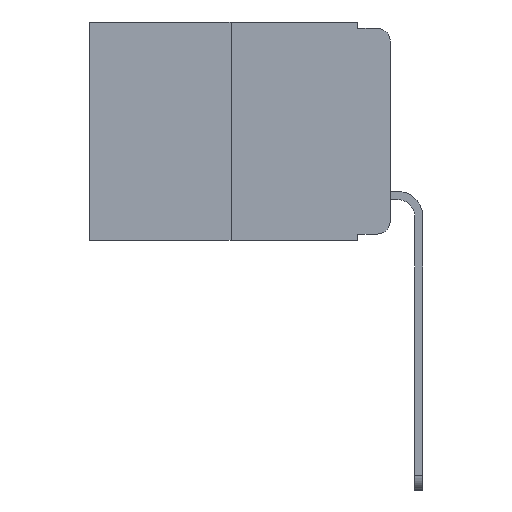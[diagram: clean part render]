
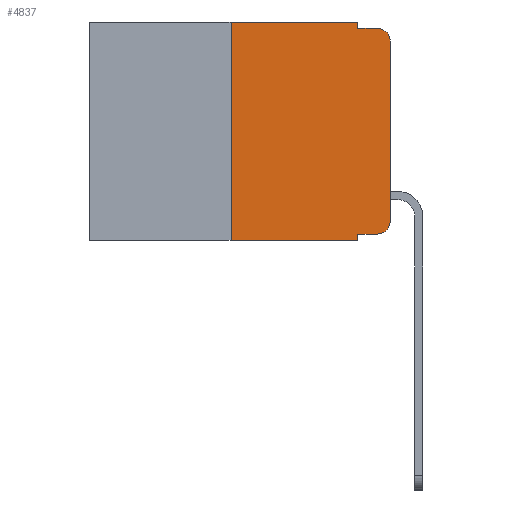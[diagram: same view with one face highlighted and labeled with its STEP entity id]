
A CAD part, left-side view. The second image highlights one B-rep face of the part: STEP entity #4837.
In plain terms, the highlighted planar face has unit normal (-1, 0, 0).
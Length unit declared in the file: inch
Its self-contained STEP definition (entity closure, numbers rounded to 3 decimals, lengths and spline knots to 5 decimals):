
#92 = CARTESIAN_POINT ( 'NONE',  ( 0., 0.02, -0.313 ) ) ;
#357 = DIRECTION ( 'NONE',  ( -1., 0., 0. ) ) ;
#649 = EDGE_CURVE ( 'NONE', #11194, #3836, #3087, .T. ) ;
#843 = CIRCLE ( 'NONE', #3029, 0.02 ) ;
#900 = CARTESIAN_POINT ( 'NONE',  ( 0., 0., -0.313 ) ) ;
#951 = CARTESIAN_POINT ( 'NONE',  ( 0., 0.051, -0.01 ) ) ;
#1226 = VECTOR ( 'NONE', #12074, 39.37008 ) ;
#1256 = LINE ( 'NONE', #2487, #8722 ) ;
#1685 = AXIS2_PLACEMENT_3D ( 'NONE', #9962, #4475, #8779 ) ;
#1732 = LINE ( 'NONE', #2476, #4293 ) ;
#1892 = CARTESIAN_POINT ( 'NONE',  ( 0., 0., -0.03 ) ) ;
#1922 = LINE ( 'NONE', #12466, #9677 ) ;
#2108 = DIRECTION ( 'NONE',  ( -1., 0., 0. ) ) ;
#2287 = ORIENTED_EDGE ( 'NONE', *, *, #12349, .F. ) ;
#2432 = ORIENTED_EDGE ( 'NONE', *, *, #12384, .F. ) ;
#2476 = CARTESIAN_POINT ( 'NONE',  ( 0., 0.051, -0.333 ) ) ;
#2487 = CARTESIAN_POINT ( 'NONE',  ( 0., 0.051, 0. ) ) ;
#2588 = CIRCLE ( 'NONE', #11765, 0.02 ) ;
#2600 = ORIENTED_EDGE ( 'NONE', *, *, #11514, .F. ) ;
#2742 = VECTOR ( 'NONE', #11522, 39.37008 ) ;
#2748 = ORIENTED_EDGE ( 'NONE', *, *, #10290, .T. ) ;
#2786 = EDGE_CURVE ( 'NONE', #12239, #5759, #843, .T. ) ;
#2811 = CARTESIAN_POINT ( 'NONE',  ( 0., 0.051, 0. ) ) ;
#2853 = DIRECTION ( 'NONE',  ( 0., -1., 0. ) ) ;
#2943 = ORIENTED_EDGE ( 'NONE', *, *, #6075, .T. ) ;
#3029 = AXIS2_PLACEMENT_3D ( 'NONE', #92, #357, #11572 ) ;
#3087 = LINE ( 'NONE', #10146, #10669 ) ;
#3102 = DIRECTION ( 'NONE',  ( 0., 0., -1. ) ) ;
#3784 = VERTEX_POINT ( 'NONE', #7944 ) ;
#3836 = VERTEX_POINT ( 'NONE', #10761 ) ;
#4117 = VECTOR ( 'NONE', #11931, 39.37008 ) ;
#4293 = VECTOR ( 'NONE', #11411, 39.37008 ) ;
#4377 = CARTESIAN_POINT ( 'NONE',  ( 0., 0.473, 0. ) ) ;
#4475 = DIRECTION ( 'NONE',  ( 1., 0., 0. ) ) ;
#4742 = VECTOR ( 'NONE', #10235, 39.37008 ) ;
#4775 = CARTESIAN_POINT ( 'NONE',  ( 0., 0.25, 0. ) ) ;
#4812 = VERTEX_POINT ( 'NONE', #1892 ) ;
#4837 = ADVANCED_FACE ( 'NONE', ( #12047 ), #11092, .F. ) ;
#5175 = VERTEX_POINT ( 'NONE', #7815 ) ;
#5425 = CARTESIAN_POINT ( 'NONE',  ( 0., 0.051, 0. ) ) ;
#5643 = VERTEX_POINT ( 'NONE', #7412 ) ;
#5759 = VERTEX_POINT ( 'NONE', #900 ) ;
#6075 = EDGE_CURVE ( 'NONE', #5759, #4812, #1922, .T. ) ;
#6651 = EDGE_CURVE ( 'NONE', #3784, #3836, #1256, .T. ) ;
#6743 = LINE ( 'NONE', #951, #4117 ) ;
#7152 = ORIENTED_EDGE ( 'NONE', *, *, #8594, .F. ) ;
#7174 = ORIENTED_EDGE ( 'NONE', *, *, #649, .T. ) ;
#7412 = CARTESIAN_POINT ( 'NONE',  ( 0., 0.051, -0.01 ) ) ;
#7558 = ORIENTED_EDGE ( 'NONE', *, *, #10623, .T. ) ;
#7672 = ORIENTED_EDGE ( 'NONE', *, *, #6651, .F. ) ;
#7815 = CARTESIAN_POINT ( 'NONE',  ( 0., 0.25, 0. ) ) ;
#7944 = CARTESIAN_POINT ( 'NONE',  ( 0., 0.051, -0.333 ) ) ;
#7966 = ORIENTED_EDGE ( 'NONE', *, *, #2786, .T. ) ;
#8213 = CARTESIAN_POINT ( 'NONE',  ( 0., 0.02, -0.03 ) ) ;
#8594 = EDGE_CURVE ( 'NONE', #11194, #5175, #9331, .T. ) ;
#8722 = VECTOR ( 'NONE', #3102, 39.37008 ) ;
#8779 = DIRECTION ( 'NONE',  ( 0., 0., -1. ) ) ;
#8876 = DIRECTION ( 'NONE',  ( 0., 0., 1. ) ) ;
#9181 = DIRECTION ( 'NONE',  ( 0., 0., -1. ) ) ;
#9331 = LINE ( 'NONE', #4775, #2742 ) ;
#9633 = LINE ( 'NONE', #5425, #1226 ) ;
#9649 = VERTEX_POINT ( 'NONE', #10049 ) ;
#9677 = VECTOR ( 'NONE', #8876, 39.37008 ) ;
#9950 = LINE ( 'NONE', #4377, #4742 ) ;
#9962 = CARTESIAN_POINT ( 'NONE',  ( 0., 0.473, 0. ) ) ;
#9985 = EDGE_LOOP ( 'NONE', ( #2943, #2748, #2600, #2432, #2287, #7152, #7174, #7672, #7558, #7966 ) ) ;
#10049 = CARTESIAN_POINT ( 'NONE',  ( 0., 0.02, -0.01 ) ) ;
#10146 = CARTESIAN_POINT ( 'NONE',  ( 0., 0.473, -0.343 ) ) ;
#10235 = DIRECTION ( 'NONE',  ( 0., -1., 0. ) ) ;
#10290 = EDGE_CURVE ( 'NONE', #4812, #9649, #2588, .T. ) ;
#10623 = EDGE_CURVE ( 'NONE', #3784, #12239, #1732, .T. ) ;
#10669 = VECTOR ( 'NONE', #2853, 39.37008 ) ;
#10761 = CARTESIAN_POINT ( 'NONE',  ( 0., 0.051, -0.343 ) ) ;
#11092 = PLANE ( 'NONE',  #1685 ) ;
#11194 = VERTEX_POINT ( 'NONE', #12007 ) ;
#11411 = DIRECTION ( 'NONE',  ( 0., -1., 0. ) ) ;
#11514 = EDGE_CURVE ( 'NONE', #5643, #9649, #6743, .T. ) ;
#11522 = DIRECTION ( 'NONE',  ( 0., 0., 1. ) ) ;
#11572 = DIRECTION ( 'NONE',  ( 0., 0., -1. ) ) ;
#11765 = AXIS2_PLACEMENT_3D ( 'NONE', #8213, #2108, #9181 ) ;
#11917 = CARTESIAN_POINT ( 'NONE',  ( 0., 0.02, -0.333 ) ) ;
#11931 = DIRECTION ( 'NONE',  ( 0., -1., 0. ) ) ;
#12007 = CARTESIAN_POINT ( 'NONE',  ( 0., 0.25, -0.343 ) ) ;
#12047 = FACE_OUTER_BOUND ( 'NONE', #9985, .T. ) ;
#12074 = DIRECTION ( 'NONE',  ( 0., 0., -1. ) ) ;
#12195 = VERTEX_POINT ( 'NONE', #2811 ) ;
#12239 = VERTEX_POINT ( 'NONE', #11917 ) ;
#12349 = EDGE_CURVE ( 'NONE', #5175, #12195, #9950, .T. ) ;
#12384 = EDGE_CURVE ( 'NONE', #12195, #5643, #9633, .T. ) ;
#12466 = CARTESIAN_POINT ( 'NONE',  ( 0., 0., 0. ) ) ;
